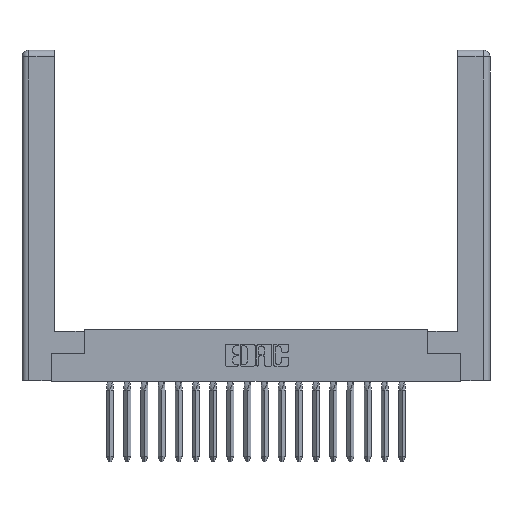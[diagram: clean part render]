
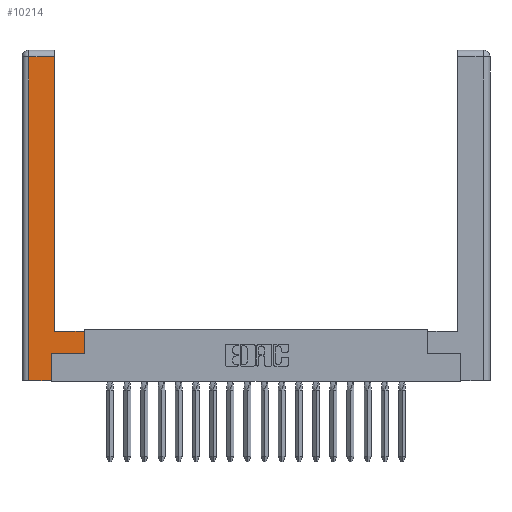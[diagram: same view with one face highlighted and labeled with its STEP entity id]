
A CAD part, top view. The second image highlights one B-rep face of the part: STEP entity #10214.
In plain terms, the highlighted planar face has unit normal (0, 0, 1).
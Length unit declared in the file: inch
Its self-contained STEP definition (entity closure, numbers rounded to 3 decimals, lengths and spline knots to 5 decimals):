
#729 = DIRECTION ( 'NONE',  ( 0., 1., 0. ) ) ;
#916 = PLANE ( 'NONE',  #2965 ) ;
#1310 = CARTESIAN_POINT ( 'NONE',  ( 0.0615, 0., 0. ) ) ;
#1506 = EDGE_CURVE ( 'NONE', #7076, #37215, #3638, .T. ) ;
#1629 = CARTESIAN_POINT ( 'NONE',  ( 0.295, 3., 0. ) ) ;
#2965 = AXIS2_PLACEMENT_3D ( 'NONE', #10070, #4030, #22524 ) ;
#3303 = ORIENTED_EDGE ( 'NONE', *, *, #9863, .T. ) ;
#3430 = VERTEX_POINT ( 'NONE', #16692 ) ;
#3638 = LINE ( 'NONE', #1310, #15598 ) ;
#4030 = DIRECTION ( 'NONE',  ( 0., 0., -1. ) ) ;
#5079 = ORIENTED_EDGE ( 'NONE', *, *, #1506, .T. ) ;
#6683 = EDGE_CURVE ( 'NONE', #15102, #3430, #32507, .T. ) ;
#6905 = CARTESIAN_POINT ( 'NONE',  ( 0.265, 0., 0. ) ) ;
#7076 = VERTEX_POINT ( 'NONE', #24042 ) ;
#7637 = EDGE_CURVE ( 'NONE', #26382, #26353, #29140, .T. ) ;
#7640 = LINE ( 'NONE', #33634, #25815 ) ;
#8096 = VECTOR ( 'NONE', #38647, 39.37008 ) ;
#8125 = VERTEX_POINT ( 'NONE', #12317 ) ;
#8188 = ORIENTED_EDGE ( 'NONE', *, *, #6683, .T. ) ;
#8656 = ORIENTED_EDGE ( 'NONE', *, *, #7637, .T. ) ;
#8993 = EDGE_CURVE ( 'NONE', #37215, #26382, #28080, .T. ) ;
#9314 = VECTOR ( 'NONE', #36930, 39.37008 ) ;
#9629 = CARTESIAN_POINT ( 'NONE',  ( 0.565, 0.245, 0. ) ) ;
#9756 = CARTESIAN_POINT ( 'NONE',  ( 0.565, 0.45, 0. ) ) ;
#9863 = EDGE_CURVE ( 'NONE', #26353, #10633, #34224, .T. ) ;
#10050 = EDGE_CURVE ( 'NONE', #8125, #15102, #17418, .T. ) ;
#10070 = CARTESIAN_POINT ( 'NONE',  ( 0., 0., 0. ) ) ;
#10214 = ADVANCED_FACE ( 'NONE', ( #24155 ), #916, .F. ) ;
#10633 = VERTEX_POINT ( 'NONE', #9629 ) ;
#10948 = VECTOR ( 'NONE', #729, 39.37008 ) ;
#12317 = CARTESIAN_POINT ( 'NONE',  ( 0.565, 0.45, 0. ) ) ;
#14249 = VECTOR ( 'NONE', #25066, 39.37008 ) ;
#15102 = VERTEX_POINT ( 'NONE', #30113 ) ;
#15598 = VECTOR ( 'NONE', #19405, 39.37008 ) ;
#16009 = VECTOR ( 'NONE', #17160, 39.37008 ) ;
#16110 = DIRECTION ( 'NONE',  ( 1., 0., 0. ) ) ;
#16692 = CARTESIAN_POINT ( 'NONE',  ( 0.295, 2.94, 0. ) ) ;
#17160 = DIRECTION ( 'NONE',  ( 1., 0., 0. ) ) ;
#17418 = LINE ( 'NONE', #24522, #9314 ) ;
#18887 = CARTESIAN_POINT ( 'NONE',  ( 0.0615, 0., 0. ) ) ;
#19405 = DIRECTION ( 'NONE',  ( 0., -1., 0. ) ) ;
#19605 = LINE ( 'NONE', #9756, #10948 ) ;
#19768 = CARTESIAN_POINT ( 'NONE',  ( 0.265, 0.245, 0. ) ) ;
#21444 = ORIENTED_EDGE ( 'NONE', *, *, #10050, .T. ) ;
#21616 = EDGE_CURVE ( 'NONE', #10633, #8125, #19605, .T. ) ;
#22204 = EDGE_CURVE ( 'NONE', #3430, #7076, #7640, .T. ) ;
#22524 = DIRECTION ( 'NONE',  ( -1., 0., 0. ) ) ;
#22576 = EDGE_LOOP ( 'NONE', ( #8188, #32944, #5079, #29920, #8656, #3303, #27752, #21444 ) ) ;
#24042 = CARTESIAN_POINT ( 'NONE',  ( 0.0615, 2.94, 0. ) ) ;
#24155 = FACE_OUTER_BOUND ( 'NONE', #22576, .T. ) ;
#24251 = VECTOR ( 'NONE', #16110, 39.37008 ) ;
#24522 = CARTESIAN_POINT ( 'NONE',  ( 0.295, 0.45, 0. ) ) ;
#25066 = DIRECTION ( 'NONE',  ( 0., 1., 0. ) ) ;
#25815 = VECTOR ( 'NONE', #36698, 39.37008 ) ;
#26353 = VERTEX_POINT ( 'NONE', #19768 ) ;
#26382 = VERTEX_POINT ( 'NONE', #35270 ) ;
#27752 = ORIENTED_EDGE ( 'NONE', *, *, #21616, .T. ) ;
#28080 = LINE ( 'NONE', #6905, #24251 ) ;
#29140 = LINE ( 'NONE', #31336, #14249 ) ;
#29920 = ORIENTED_EDGE ( 'NONE', *, *, #8993, .T. ) ;
#30113 = CARTESIAN_POINT ( 'NONE',  ( 0.295, 0.45, 0. ) ) ;
#31336 = CARTESIAN_POINT ( 'NONE',  ( 0.265, 0.245, 0. ) ) ;
#32507 = LINE ( 'NONE', #1629, #8096 ) ;
#32944 = ORIENTED_EDGE ( 'NONE', *, *, #22204, .T. ) ;
#33634 = CARTESIAN_POINT ( 'NONE',  ( 0.0615, 2.94, 0. ) ) ;
#34224 = LINE ( 'NONE', #38916, #16009 ) ;
#35270 = CARTESIAN_POINT ( 'NONE',  ( 0.265, 0., 0. ) ) ;
#36698 = DIRECTION ( 'NONE',  ( -1., 0., 0. ) ) ;
#36930 = DIRECTION ( 'NONE',  ( -1., 0., 0. ) ) ;
#37215 = VERTEX_POINT ( 'NONE', #18887 ) ;
#38647 = DIRECTION ( 'NONE',  ( 0., 1., 0. ) ) ;
#38916 = CARTESIAN_POINT ( 'NONE',  ( 0.565, 0.245, 0. ) ) ;
